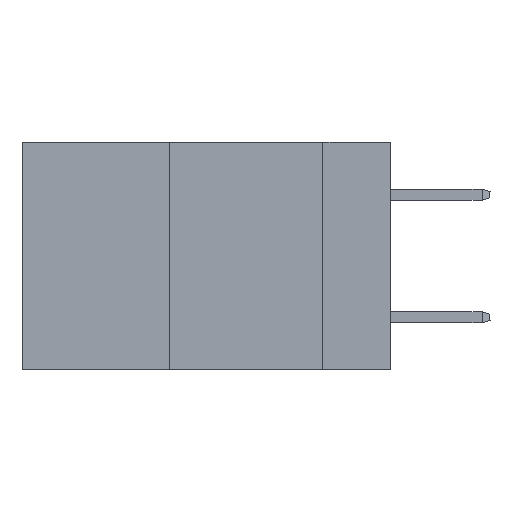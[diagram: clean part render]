
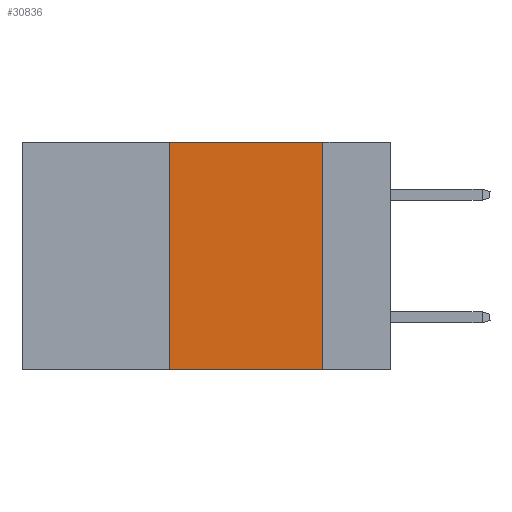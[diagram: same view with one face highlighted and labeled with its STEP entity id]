
A CAD part, left-side view. The second image highlights one B-rep face of the part: STEP entity #30836.
In plain terms, the highlighted planar face has unit normal (-1, 0, 0).
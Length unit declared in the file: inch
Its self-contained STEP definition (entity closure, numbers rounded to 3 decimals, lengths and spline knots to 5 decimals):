
#203 = FACE_OUTER_BOUND ( 'NONE', #7697, .T. ) ;
#3168 = CARTESIAN_POINT ( 'NONE',  ( 0., 0.36, -0.37 ) ) ;
#4569 = EDGE_CURVE ( 'NONE', #26947, #6033, #14004, .T. ) ;
#5545 = CARTESIAN_POINT ( 'NONE',  ( 0., 0.6, 0. ) ) ;
#5871 = CARTESIAN_POINT ( 'NONE',  ( 0., 0.11, 0. ) ) ;
#6033 = VERTEX_POINT ( 'NONE', #12741 ) ;
#6916 = VECTOR ( 'NONE', #35248, 39.37008 ) ;
#7100 = ORIENTED_EDGE ( 'NONE', *, *, #23688, .F. ) ;
#7697 = EDGE_LOOP ( 'NONE', ( #15651, #28418, #7100, #24222 ) ) ;
#10052 = VECTOR ( 'NONE', #23745, 39.37008 ) ;
#10627 = VERTEX_POINT ( 'NONE', #10732 ) ;
#10732 = CARTESIAN_POINT ( 'NONE',  ( 0., 0.36, 0. ) ) ;
#10825 = EDGE_CURVE ( 'NONE', #10627, #25218, #19124, .T. ) ;
#12741 = CARTESIAN_POINT ( 'NONE',  ( 0., 0.11, -0.37 ) ) ;
#12869 = PLANE ( 'NONE',  #22841 ) ;
#14004 = LINE ( 'NONE', #30344, #29134 ) ;
#15651 = ORIENTED_EDGE ( 'NONE', *, *, #38879, .F. ) ;
#15943 = CARTESIAN_POINT ( 'NONE',  ( 0., 0.6, 0. ) ) ;
#19016 = DIRECTION ( 'NONE',  ( 0., 0., -1. ) ) ;
#19124 = LINE ( 'NONE', #5545, #10052 ) ;
#20427 = CARTESIAN_POINT ( 'NONE',  ( 0., 0.11, 0. ) ) ;
#22841 = AXIS2_PLACEMENT_3D ( 'NONE', #15943, #36845, #19016 ) ;
#23688 = EDGE_CURVE ( 'NONE', #26947, #10627, #36103, .T. ) ;
#23745 = DIRECTION ( 'NONE',  ( 0., -1., 0. ) ) ;
#24222 = ORIENTED_EDGE ( 'NONE', *, *, #4569, .T. ) ;
#25218 = VERTEX_POINT ( 'NONE', #5871 ) ;
#26170 = DIRECTION ( 'NONE',  ( 0., 0., 1. ) ) ;
#26416 = VECTOR ( 'NONE', #26170, 39.37008 ) ;
#26947 = VERTEX_POINT ( 'NONE', #3168 ) ;
#28418 = ORIENTED_EDGE ( 'NONE', *, *, #10825, .F. ) ;
#29134 = VECTOR ( 'NONE', #33321, 39.37008 ) ;
#30344 = CARTESIAN_POINT ( 'NONE',  ( 0., 0.6, -0.37 ) ) ;
#30836 = ADVANCED_FACE ( 'NONE', ( #203 ), #12869, .F. ) ;
#31038 = LINE ( 'NONE', #20427, #6916 ) ;
#33321 = DIRECTION ( 'NONE',  ( 0., -1., 0. ) ) ;
#34934 = CARTESIAN_POINT ( 'NONE',  ( 0., 0.36, 0. ) ) ;
#35248 = DIRECTION ( 'NONE',  ( 0., 0., -1. ) ) ;
#36103 = LINE ( 'NONE', #34934, #26416 ) ;
#36845 = DIRECTION ( 'NONE',  ( 1., 0., 0. ) ) ;
#38879 = EDGE_CURVE ( 'NONE', #25218, #6033, #31038, .T. ) ;
